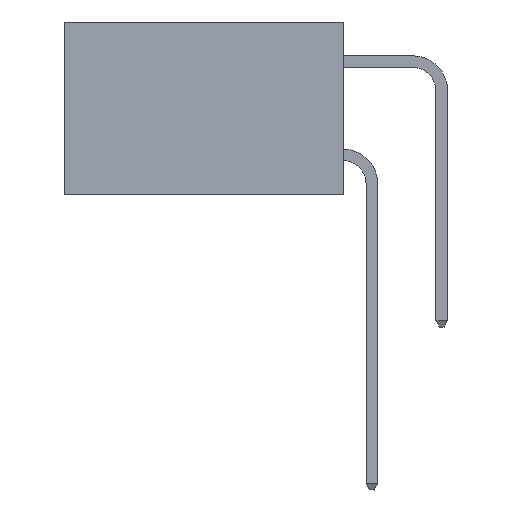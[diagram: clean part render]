
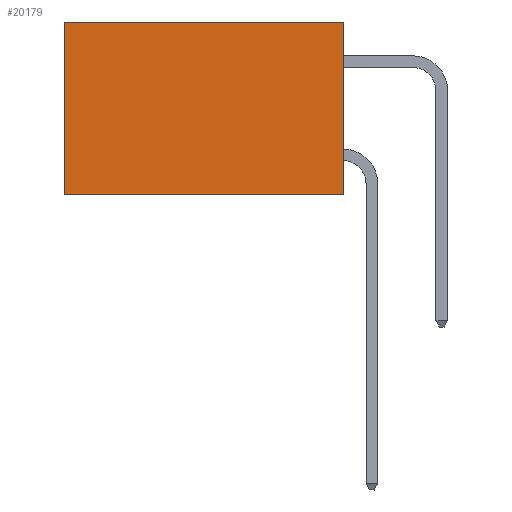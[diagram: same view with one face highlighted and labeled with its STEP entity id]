
A CAD part, left-side view. The second image highlights one B-rep face of the part: STEP entity #20179.
In plain terms, the highlighted planar face has unit normal (-1, 0, 0).
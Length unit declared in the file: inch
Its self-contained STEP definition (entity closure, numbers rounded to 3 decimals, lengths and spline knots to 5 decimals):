
#166 = LINE ( 'NONE', #18138, #17023 ) ;
#1119 = LINE ( 'NONE', #10114, #9103 ) ;
#3429 = LINE ( 'NONE', #12013, #24137 ) ;
#3524 = EDGE_CURVE ( 'NONE', #24728, #8862, #3429, .T. ) ;
#3940 = DIRECTION ( 'NONE',  ( 0., 0., -1. ) ) ;
#5271 = DIRECTION ( 'NONE',  ( 0., 1., 0. ) ) ;
#5363 = CARTESIAN_POINT ( 'NONE',  ( 0.298, 0., -0.37 ) ) ;
#5679 = PLANE ( 'NONE',  #8398 ) ;
#5856 = DIRECTION ( 'NONE',  ( 1., 0., 0. ) ) ;
#6296 = DIRECTION ( 'NONE',  ( 0., 0., -1. ) ) ;
#7752 = DIRECTION ( 'NONE',  ( 0., 1., 0. ) ) ;
#8398 = AXIS2_PLACEMENT_3D ( 'NONE', #19993, #5856, #23922 ) ;
#8862 = VERTEX_POINT ( 'NONE', #19274 ) ;
#9103 = VECTOR ( 'NONE', #3940, 39.37008 ) ;
#9476 = ORIENTED_EDGE ( 'NONE', *, *, #11769, .T. ) ;
#9504 = EDGE_CURVE ( 'NONE', #13269, #13668, #18110, .T. ) ;
#10114 = CARTESIAN_POINT ( 'NONE',  ( 0.298, 0.6, 0. ) ) ;
#10421 = EDGE_LOOP ( 'NONE', ( #9476, #15809, #11200, #20421 ) ) ;
#11200 = ORIENTED_EDGE ( 'NONE', *, *, #26092, .F. ) ;
#11769 = EDGE_CURVE ( 'NONE', #13668, #8862, #1119, .T. ) ;
#12013 = CARTESIAN_POINT ( 'NONE',  ( 0.298, 0., -0.37 ) ) ;
#13269 = VERTEX_POINT ( 'NONE', #25399 ) ;
#13668 = VERTEX_POINT ( 'NONE', #20945 ) ;
#15809 = ORIENTED_EDGE ( 'NONE', *, *, #3524, .F. ) ;
#17023 = VECTOR ( 'NONE', #6296, 39.37008 ) ;
#18110 = LINE ( 'NONE', #24609, #23832 ) ;
#18138 = CARTESIAN_POINT ( 'NONE',  ( 0.298, 0., 0. ) ) ;
#19274 = CARTESIAN_POINT ( 'NONE',  ( 0.298, 0.6, -0.37 ) ) ;
#19993 = CARTESIAN_POINT ( 'NONE',  ( 0.298, 0., 0. ) ) ;
#20179 = ADVANCED_FACE ( 'NONE', ( #21840 ), #5679, .F. ) ;
#20421 = ORIENTED_EDGE ( 'NONE', *, *, #9504, .T. ) ;
#20945 = CARTESIAN_POINT ( 'NONE',  ( 0.298, 0.6, 0. ) ) ;
#21840 = FACE_OUTER_BOUND ( 'NONE', #10421, .T. ) ;
#23832 = VECTOR ( 'NONE', #5271, 39.37008 ) ;
#23922 = DIRECTION ( 'NONE',  ( 0., 0., -1. ) ) ;
#24137 = VECTOR ( 'NONE', #7752, 39.37008 ) ;
#24609 = CARTESIAN_POINT ( 'NONE',  ( 0.298, 0., 0. ) ) ;
#24728 = VERTEX_POINT ( 'NONE', #5363 ) ;
#25399 = CARTESIAN_POINT ( 'NONE',  ( 0.298, 0., 0. ) ) ;
#26092 = EDGE_CURVE ( 'NONE', #13269, #24728, #166, .T. ) ;
